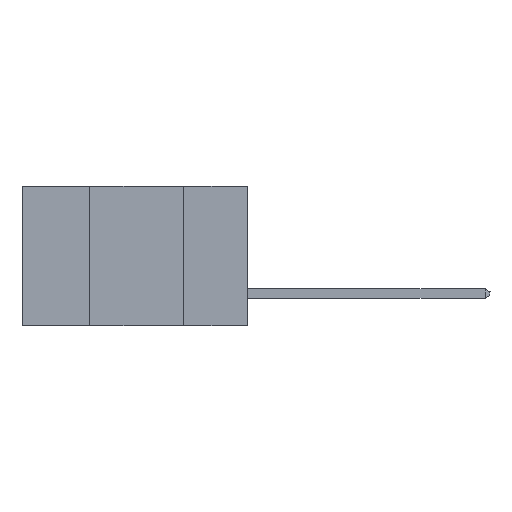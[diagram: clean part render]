
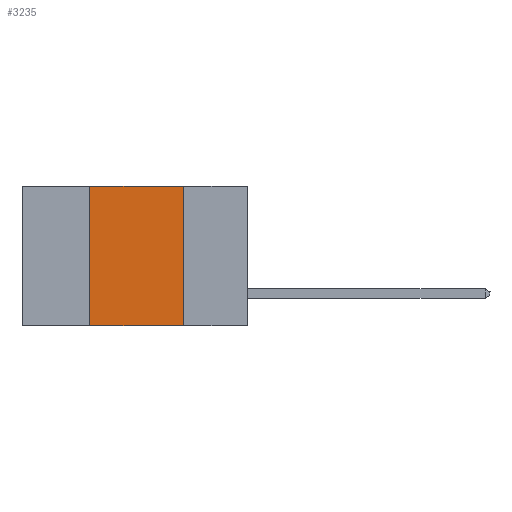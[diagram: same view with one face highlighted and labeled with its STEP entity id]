
A CAD part, left-side view. The second image highlights one B-rep face of the part: STEP entity #3235.
In plain terms, the highlighted planar face has unit normal (-1, 0, 0).
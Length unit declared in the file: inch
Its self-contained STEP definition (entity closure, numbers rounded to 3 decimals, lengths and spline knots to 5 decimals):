
#339 = VERTEX_POINT ( 'NONE', #4983 ) ;
#1074 = CARTESIAN_POINT ( 'NONE',  ( 0., 0.42, 0. ) ) ;
#1439 = VECTOR ( 'NONE', #8479, 39.37008 ) ;
#1578 = CARTESIAN_POINT ( 'NONE',  ( 0., 0.6, 0. ) ) ;
#2104 = CARTESIAN_POINT ( 'NONE',  ( 0., 0.17, -0.37 ) ) ;
#2355 = CARTESIAN_POINT ( 'NONE',  ( 0., 0.42, -0.37 ) ) ;
#2489 = VECTOR ( 'NONE', #7099, 39.37008 ) ;
#2776 = VERTEX_POINT ( 'NONE', #8046 ) ;
#2974 = CARTESIAN_POINT ( 'NONE',  ( 0., 0.6, -0.37 ) ) ;
#3235 = ADVANCED_FACE ( 'NONE', ( #10364 ), #7945, .F. ) ;
#3885 = DIRECTION ( 'NONE',  ( 0., 0., -1. ) ) ;
#4319 = EDGE_CURVE ( 'NONE', #2776, #8991, #10637, .T. ) ;
#4983 = CARTESIAN_POINT ( 'NONE',  ( 0., 0.17, 0. ) ) ;
#5047 = CARTESIAN_POINT ( 'NONE',  ( 0., 0.6, 0. ) ) ;
#5122 = CARTESIAN_POINT ( 'NONE',  ( 0., 0.17, -0.37 ) ) ;
#5404 = EDGE_CURVE ( 'NONE', #339, #8991, #12249, .T. ) ;
#5612 = VECTOR ( 'NONE', #12101, 39.37008 ) ;
#7099 = DIRECTION ( 'NONE',  ( 0., 0., 1. ) ) ;
#7327 = EDGE_LOOP ( 'NONE', ( #11325, #9799, #13621, #8399 ) ) ;
#7621 = AXIS2_PLACEMENT_3D ( 'NONE', #1578, #12169, #3885 ) ;
#7679 = LINE ( 'NONE', #2355, #2489 ) ;
#7945 = PLANE ( 'NONE',  #7621 ) ;
#7950 = EDGE_CURVE ( 'NONE', #2776, #8968, #7679, .T. ) ;
#8046 = CARTESIAN_POINT ( 'NONE',  ( 0., 0.42, -0.37 ) ) ;
#8399 = ORIENTED_EDGE ( 'NONE', *, *, #4319, .T. ) ;
#8479 = DIRECTION ( 'NONE',  ( 0., -1., 0. ) ) ;
#8968 = VERTEX_POINT ( 'NONE', #1074 ) ;
#8991 = VERTEX_POINT ( 'NONE', #2104 ) ;
#9326 = DIRECTION ( 'NONE',  ( 0., -1., 0. ) ) ;
#9799 = ORIENTED_EDGE ( 'NONE', *, *, #10413, .F. ) ;
#10364 = FACE_OUTER_BOUND ( 'NONE', #7327, .T. ) ;
#10413 = EDGE_CURVE ( 'NONE', #8968, #339, #11309, .T. ) ;
#10637 = LINE ( 'NONE', #2974, #12486 ) ;
#11309 = LINE ( 'NONE', #5047, #1439 ) ;
#11325 = ORIENTED_EDGE ( 'NONE', *, *, #5404, .F. ) ;
#12101 = DIRECTION ( 'NONE',  ( 0., 0., -1. ) ) ;
#12169 = DIRECTION ( 'NONE',  ( 1., 0., 0. ) ) ;
#12249 = LINE ( 'NONE', #5122, #5612 ) ;
#12486 = VECTOR ( 'NONE', #9326, 39.37008 ) ;
#13621 = ORIENTED_EDGE ( 'NONE', *, *, #7950, .F. ) ;
